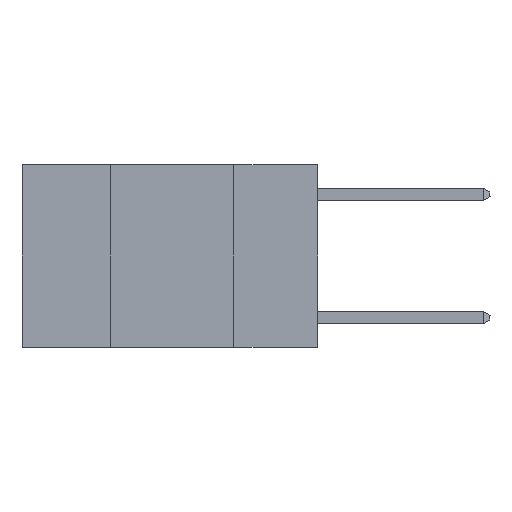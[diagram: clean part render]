
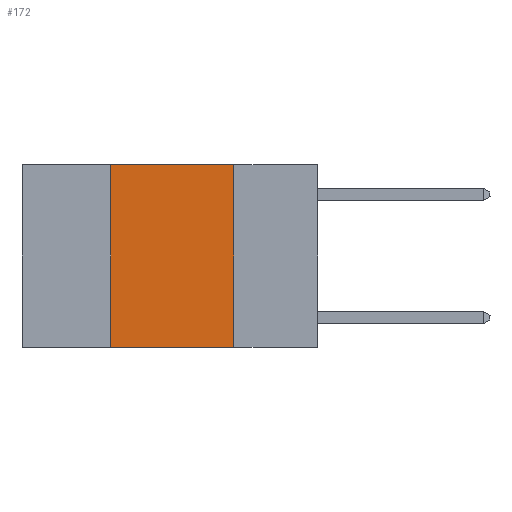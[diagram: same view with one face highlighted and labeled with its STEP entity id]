
A CAD part, left-side view. The second image highlights one B-rep face of the part: STEP entity #172.
In plain terms, the highlighted planar face has unit normal (-1, 0, 0).
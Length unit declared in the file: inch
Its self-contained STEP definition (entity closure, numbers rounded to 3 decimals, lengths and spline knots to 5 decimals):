
#152 = LINE ( 'NONE', #9233, #1536 ) ;
#172 = ADVANCED_FACE ( 'NONE', ( #2822 ), #7177, .F. ) ;
#678 = ORIENTED_EDGE ( 'NONE', *, *, #2968, .T. ) ;
#1015 = DIRECTION ( 'NONE',  ( 0., 0., 1. ) ) ;
#1297 = ORIENTED_EDGE ( 'NONE', *, *, #2838, .F. ) ;
#1345 = EDGE_LOOP ( 'NONE', ( #1297, #9379, #9244, #678 ) ) ;
#1536 = VECTOR ( 'NONE', #4590, 39.37008 ) ;
#2670 = CARTESIAN_POINT ( 'NONE',  ( 0., 0.17, 0. ) ) ;
#2822 = FACE_OUTER_BOUND ( 'NONE', #1345, .T. ) ;
#2838 = EDGE_CURVE ( 'NONE', #7394, #3492, #3499, .T. ) ;
#2968 = EDGE_CURVE ( 'NONE', #10707, #3492, #5153, .T. ) ;
#3492 = VERTEX_POINT ( 'NONE', #11611 ) ;
#3499 = LINE ( 'NONE', #2670, #8869 ) ;
#4590 = DIRECTION ( 'NONE',  ( 0., -1., 0. ) ) ;
#4777 = CARTESIAN_POINT ( 'NONE',  ( 0., 0.42, 0. ) ) ;
#5153 = LINE ( 'NONE', #8828, #10795 ) ;
#5198 = CARTESIAN_POINT ( 'NONE',  ( 0., 0.42, -0.37 ) ) ;
#5448 = EDGE_CURVE ( 'NONE', #10707, #7854, #11712, .T. ) ;
#5650 = CARTESIAN_POINT ( 'NONE',  ( 0., 0.42, 0. ) ) ;
#5766 = EDGE_CURVE ( 'NONE', #7854, #7394, #152, .T. ) ;
#5816 = DIRECTION ( 'NONE',  ( 0., 0., -1. ) ) ;
#7177 = PLANE ( 'NONE',  #9714 ) ;
#7394 = VERTEX_POINT ( 'NONE', #10924 ) ;
#7854 = VERTEX_POINT ( 'NONE', #5650 ) ;
#8828 = CARTESIAN_POINT ( 'NONE',  ( 0., 0.6, -0.37 ) ) ;
#8869 = VECTOR ( 'NONE', #10708, 39.37008 ) ;
#9034 = VECTOR ( 'NONE', #1015, 39.37008 ) ;
#9233 = CARTESIAN_POINT ( 'NONE',  ( 0., 0.6, 0. ) ) ;
#9244 = ORIENTED_EDGE ( 'NONE', *, *, #5448, .F. ) ;
#9379 = ORIENTED_EDGE ( 'NONE', *, *, #5766, .F. ) ;
#9714 = AXIS2_PLACEMENT_3D ( 'NONE', #9950, #10364, #5816 ) ;
#9746 = DIRECTION ( 'NONE',  ( 0., -1., 0. ) ) ;
#9950 = CARTESIAN_POINT ( 'NONE',  ( 0., 0.6, 0. ) ) ;
#10364 = DIRECTION ( 'NONE',  ( 1., 0., 0. ) ) ;
#10707 = VERTEX_POINT ( 'NONE', #5198 ) ;
#10708 = DIRECTION ( 'NONE',  ( 0., 0., -1. ) ) ;
#10795 = VECTOR ( 'NONE', #9746, 39.37008 ) ;
#10924 = CARTESIAN_POINT ( 'NONE',  ( 0., 0.17, 0. ) ) ;
#11611 = CARTESIAN_POINT ( 'NONE',  ( 0., 0.17, -0.37 ) ) ;
#11712 = LINE ( 'NONE', #4777, #9034 ) ;
